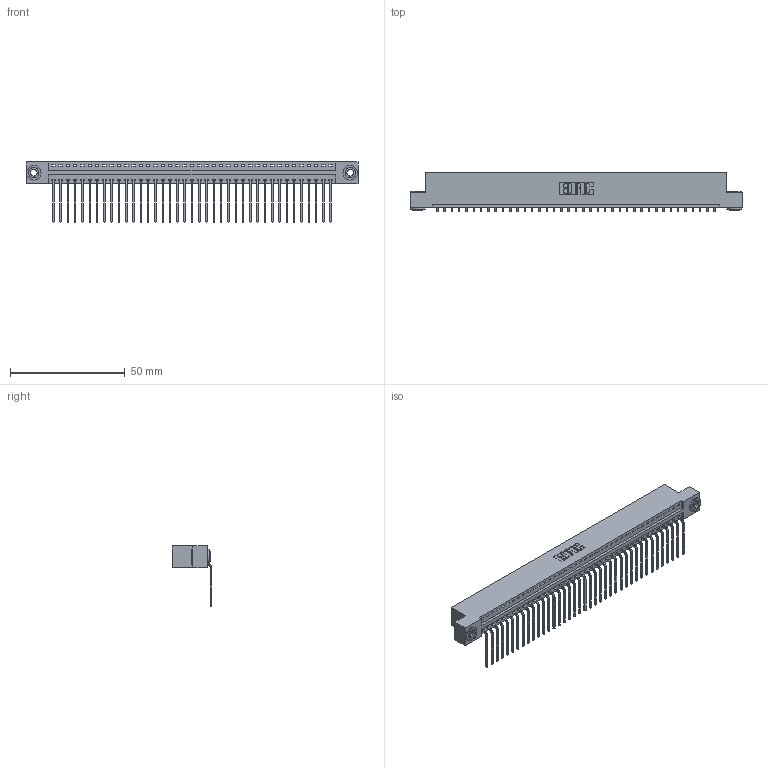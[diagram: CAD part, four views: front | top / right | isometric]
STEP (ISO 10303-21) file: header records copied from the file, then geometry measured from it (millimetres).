
FILE_DESCRIPTION (( 'STEP AP203' ), '1' );
FILE_NAME ('346-039-559-103.STEP', '2022-05-07T08:06:10', ( '' ), ( '' ), 'SwSTEP 2.0', 'SolidWorks 2020', '' );
FILE_SCHEMA (( 'CONFIG_CONTROL_DESIGN' ));
Length unit declared in the file: inch
Products named in the file (4): 345-250-002_345-250-002-102; 346-039-559-103; 345-292-001_558 559 Tail - 1; 346 Part_Flush Mounting Lugs - 0.156 Dia-TH
Assembly tree (42 placements, depth 2):
  346-039-559-103
    346 Part_Flush Mounting Lugs - 0.156 Dia-TH
    345-292-001_558 559 Tail - 1  x39
    345-250-002_345-250-002-102  x2
Bounding box: 144.4 x 17.08 x 26.16 mm (x, y, z)
Volume: 13932.7 mm3; surface area: 18408.4 mm2
Topology: 42 solids, 42 shells, 2514 faces, 7539 edges, 4970 vertices
Faces by surface type: plane 1738, cylinder 768, cone 8
Entity records: 25758 total; most frequent: CARTESIAN_POINT 4398, ORIENTED_EDGE 4362, DIRECTION 3913, EDGE_CURVE 2181, VECTOR 1869, LINE 1869, VERTEX_POINT 1450, AXIS2_PLACEMENT_3D 1022
